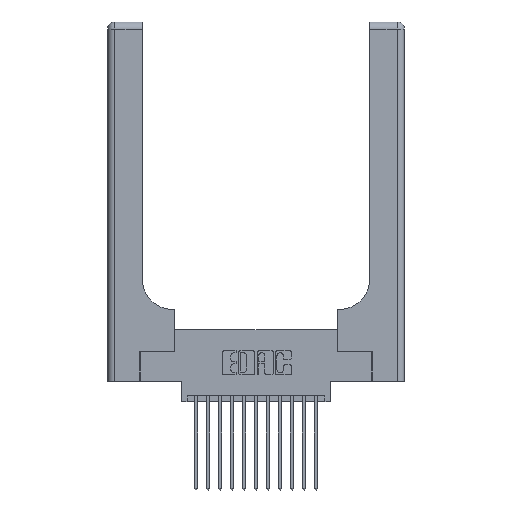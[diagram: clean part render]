
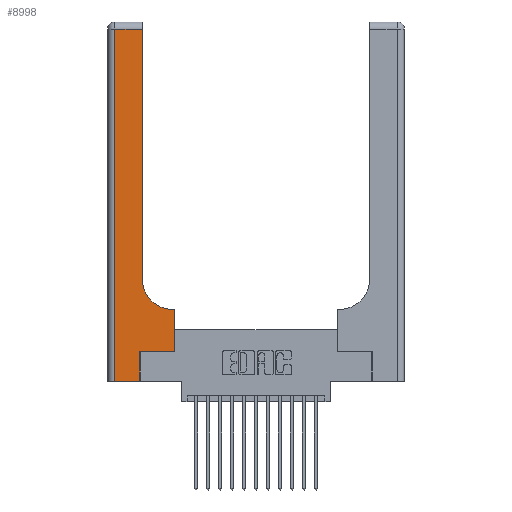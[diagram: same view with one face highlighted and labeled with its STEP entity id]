
A CAD part, top view. The second image highlights one B-rep face of the part: STEP entity #8998.
In plain terms, the highlighted planar face has unit normal (0, 0, 1).
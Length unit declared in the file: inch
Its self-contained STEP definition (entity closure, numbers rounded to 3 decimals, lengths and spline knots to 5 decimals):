
#44 = CARTESIAN_POINT ( 'NONE',  ( 0.06, 0., 0.37 ) ) ;
#663 = ORIENTED_EDGE ( 'NONE', *, *, #17998, .T. ) ;
#926 = DIRECTION ( 'NONE',  ( -1., 0., 0. ) ) ;
#936 = CARTESIAN_POINT ( 'NONE',  ( 0.2915, 0.85, 0.37 ) ) ;
#1348 = CARTESIAN_POINT ( 'NONE',  ( 0.5585, 0.6, 0.37 ) ) ;
#1401 = CARTESIAN_POINT ( 'NONE',  ( 0.269, 0., 0.37 ) ) ;
#1735 = LINE ( 'NONE', #8429, #2196 ) ;
#1851 = EDGE_CURVE ( 'NONE', #11597, #12972, #13357, .T. ) ;
#1869 = DIRECTION ( 'NONE',  ( 0., 1., 0. ) ) ;
#2029 = DIRECTION ( 'NONE',  ( 0., 0., -1. ) ) ;
#2196 = VECTOR ( 'NONE', #7002, 39.37008 ) ;
#3442 = LINE ( 'NONE', #10950, #17730 ) ;
#3549 = DIRECTION ( 'NONE',  ( 1., 0., 0. ) ) ;
#3878 = VERTEX_POINT ( 'NONE', #1348 ) ;
#4192 = VERTEX_POINT ( 'NONE', #44 ) ;
#4569 = AXIS2_PLACEMENT_3D ( 'NONE', #5586, #15325, #7028 ) ;
#4581 = CARTESIAN_POINT ( 'NONE',  ( 0.5585, 0.25, 0.37 ) ) ;
#4829 = EDGE_CURVE ( 'NONE', #4192, #11597, #1735, .T. ) ;
#4872 = CARTESIAN_POINT ( 'NONE',  ( 0.5585, 0.25, 0.37 ) ) ;
#5586 = CARTESIAN_POINT ( 'NONE',  ( 0.5415, 0.85, 0.37 ) ) ;
#5703 = ORIENTED_EDGE ( 'NONE', *, *, #16276, .T. ) ;
#5980 = EDGE_LOOP ( 'NONE', ( #14468, #12956, #10548, #9244, #12500, #663, #5703, #10759, #15488 ) ) ;
#6362 = PLANE ( 'NONE',  #10689 ) ;
#6372 = DIRECTION ( 'NONE',  ( 0., 1., 0. ) ) ;
#6645 = LINE ( 'NONE', #12019, #10383 ) ;
#7002 = DIRECTION ( 'NONE',  ( 1., 0., 0. ) ) ;
#7028 = DIRECTION ( 'NONE',  ( 1., 0., 0. ) ) ;
#7117 = EDGE_CURVE ( 'NONE', #15445, #13840, #3442, .T. ) ;
#7155 = LINE ( 'NONE', #16792, #17617 ) ;
#8080 = FACE_OUTER_BOUND ( 'NONE', #5980, .T. ) ;
#8264 = LINE ( 'NONE', #13321, #16000 ) ;
#8429 = CARTESIAN_POINT ( 'NONE',  ( 0., 0., 0.37 ) ) ;
#8641 = DIRECTION ( 'NONE',  ( 0., -1., 0. ) ) ;
#8998 = ADVANCED_FACE ( 'NONE', ( #8080 ), #6362, .F. ) ;
#9244 = ORIENTED_EDGE ( 'NONE', *, *, #4829, .T. ) ;
#9801 = VECTOR ( 'NONE', #15121, 39.37008 ) ;
#10088 = CARTESIAN_POINT ( 'NONE',  ( 0.5415, 0.6, 0.37 ) ) ;
#10202 = LINE ( 'NONE', #4872, #13875 ) ;
#10275 = EDGE_CURVE ( 'NONE', #11669, #15926, #10909, .T. ) ;
#10383 = VECTOR ( 'NONE', #3549, 39.37008 ) ;
#10548 = ORIENTED_EDGE ( 'NONE', *, *, #16649, .T. ) ;
#10594 = CARTESIAN_POINT ( 'NONE',  ( 0., 3., 0.37 ) ) ;
#10687 = LINE ( 'NONE', #17685, #9801 ) ;
#10689 = AXIS2_PLACEMENT_3D ( 'NONE', #10594, #2029, #11986 ) ;
#10759 = ORIENTED_EDGE ( 'NONE', *, *, #14888, .T. ) ;
#10909 = CIRCLE ( 'NONE', #4569, 0.25 ) ;
#10950 = CARTESIAN_POINT ( 'NONE',  ( 0., 2.94, 0.37 ) ) ;
#11597 = VERTEX_POINT ( 'NONE', #17894 ) ;
#11669 = VERTEX_POINT ( 'NONE', #10088 ) ;
#11882 = CARTESIAN_POINT ( 'NONE',  ( 0.269, 0.25, 0.37 ) ) ;
#11986 = DIRECTION ( 'NONE',  ( -1., 0., 0. ) ) ;
#12019 = CARTESIAN_POINT ( 'NONE',  ( 0.269, 0.25, 0.37 ) ) ;
#12500 = ORIENTED_EDGE ( 'NONE', *, *, #1851, .T. ) ;
#12825 = VERTEX_POINT ( 'NONE', #4581 ) ;
#12956 = ORIENTED_EDGE ( 'NONE', *, *, #7117, .T. ) ;
#12972 = VERTEX_POINT ( 'NONE', #11882 ) ;
#13242 = DIRECTION ( 'NONE',  ( 0., 1., 0. ) ) ;
#13321 = CARTESIAN_POINT ( 'NONE',  ( 0.2915, 3., 0.37 ) ) ;
#13357 = LINE ( 'NONE', #1401, #16907 ) ;
#13840 = VERTEX_POINT ( 'NONE', #13960 ) ;
#13875 = VECTOR ( 'NONE', #13242, 39.37008 ) ;
#13935 = CARTESIAN_POINT ( 'NONE',  ( 0.2915, 2.94, 0.37 ) ) ;
#13960 = CARTESIAN_POINT ( 'NONE',  ( 0.06, 2.94, 0.37 ) ) ;
#14468 = ORIENTED_EDGE ( 'NONE', *, *, #15713, .T. ) ;
#14888 = EDGE_CURVE ( 'NONE', #3878, #11669, #10687, .T. ) ;
#15121 = DIRECTION ( 'NONE',  ( -1., 0., 0. ) ) ;
#15325 = DIRECTION ( 'NONE',  ( 0., 0., -1. ) ) ;
#15445 = VERTEX_POINT ( 'NONE', #13935 ) ;
#15488 = ORIENTED_EDGE ( 'NONE', *, *, #10275, .T. ) ;
#15713 = EDGE_CURVE ( 'NONE', #15926, #15445, #8264, .T. ) ;
#15926 = VERTEX_POINT ( 'NONE', #936 ) ;
#16000 = VECTOR ( 'NONE', #6372, 39.37008 ) ;
#16276 = EDGE_CURVE ( 'NONE', #12825, #3878, #10202, .T. ) ;
#16649 = EDGE_CURVE ( 'NONE', #13840, #4192, #7155, .T. ) ;
#16792 = CARTESIAN_POINT ( 'NONE',  ( 0.06, 3., 0.37 ) ) ;
#16907 = VECTOR ( 'NONE', #1869, 39.37008 ) ;
#17617 = VECTOR ( 'NONE', #8641, 39.37008 ) ;
#17685 = CARTESIAN_POINT ( 'NONE',  ( 0.2915, 0.6, 0.37 ) ) ;
#17730 = VECTOR ( 'NONE', #926, 39.37008 ) ;
#17894 = CARTESIAN_POINT ( 'NONE',  ( 0.269, 0., 0.37 ) ) ;
#17998 = EDGE_CURVE ( 'NONE', #12972, #12825, #6645, .T. ) ;
